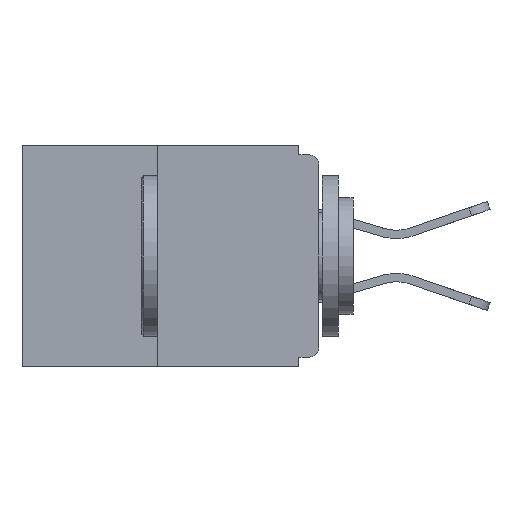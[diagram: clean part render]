
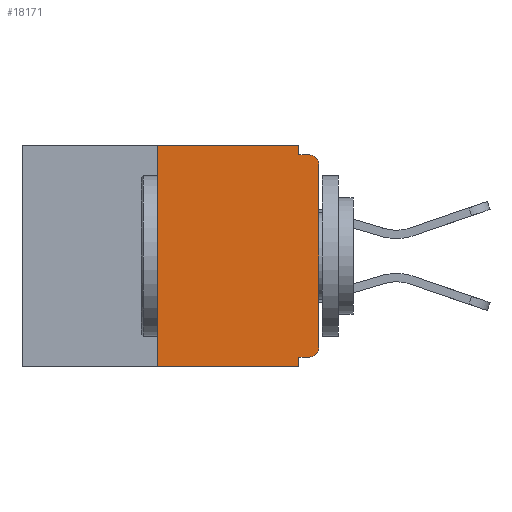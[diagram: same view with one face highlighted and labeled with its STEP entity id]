
A CAD part, left-side view. The second image highlights one B-rep face of the part: STEP entity #18171.
In plain terms, the highlighted planar face has unit normal (-1, 0, 0).
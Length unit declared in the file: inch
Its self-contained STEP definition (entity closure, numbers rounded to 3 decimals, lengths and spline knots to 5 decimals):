
#188 = CARTESIAN_POINT ( 'NONE',  ( 0., 0.031, 0. ) ) ;
#267 = DIRECTION ( 'NONE',  ( 0., 0., -1. ) ) ;
#459 = VECTOR ( 'NONE', #1966, 39.37008 ) ;
#1002 = VECTOR ( 'NONE', #4238, 39.37008 ) ;
#1060 = CARTESIAN_POINT ( 'NONE',  ( 0., 0., -0.015 ) ) ;
#1372 = CARTESIAN_POINT ( 'NONE',  ( 0., 0.46, -0.343 ) ) ;
#1966 = DIRECTION ( 'NONE',  ( 0., 0., 1. ) ) ;
#2070 = LINE ( 'NONE', #188, #21133 ) ;
#3008 = ORIENTED_EDGE ( 'NONE', *, *, #12980, .F. ) ;
#3172 = CARTESIAN_POINT ( 'NONE',  ( 0., 0.015, -0.313 ) ) ;
#3234 = DIRECTION ( 'NONE',  ( 0., 0., -1. ) ) ;
#3238 = CARTESIAN_POINT ( 'NONE',  ( 0., 0., 0. ) ) ;
#3423 = DIRECTION ( 'NONE',  ( -1., 0., 0. ) ) ;
#3539 = CARTESIAN_POINT ( 'NONE',  ( 0., 0.25, 0. ) ) ;
#3626 = CARTESIAN_POINT ( 'NONE',  ( 0., 0.25, 0. ) ) ;
#3891 = CARTESIAN_POINT ( 'NONE',  ( 0., 0.015, -0.328 ) ) ;
#4238 = DIRECTION ( 'NONE',  ( 0., -1., 0. ) ) ;
#4865 = VERTEX_POINT ( 'NONE', #9185 ) ;
#5002 = ORIENTED_EDGE ( 'NONE', *, *, #10056, .T. ) ;
#5117 = CARTESIAN_POINT ( 'NONE',  ( 0., 0.46, 0. ) ) ;
#5197 = CARTESIAN_POINT ( 'NONE',  ( 0., 0.031, -0.343 ) ) ;
#5343 = CARTESIAN_POINT ( 'NONE',  ( 0., 0.015, -0.03 ) ) ;
#6020 = EDGE_CURVE ( 'NONE', #9467, #15765, #13170, .T. ) ;
#6100 = VERTEX_POINT ( 'NONE', #13608 ) ;
#6797 = AXIS2_PLACEMENT_3D ( 'NONE', #5343, #9491, #20783 ) ;
#7282 = EDGE_CURVE ( 'NONE', #18928, #17246, #21570, .T. ) ;
#7414 = LINE ( 'NONE', #3238, #459 ) ;
#7417 = CARTESIAN_POINT ( 'NONE',  ( 0., 0., -0.03 ) ) ;
#8453 = EDGE_CURVE ( 'NONE', #17246, #20941, #2070, .T. ) ;
#8653 = ORIENTED_EDGE ( 'NONE', *, *, #7282, .F. ) ;
#8741 = CARTESIAN_POINT ( 'NONE',  ( 0., 0.015, -0.015 ) ) ;
#8863 = DIRECTION ( 'NONE',  ( 0., -1., 0. ) ) ;
#9185 = CARTESIAN_POINT ( 'NONE',  ( 0., 0., -0.313 ) ) ;
#9467 = VERTEX_POINT ( 'NONE', #7417 ) ;
#9491 = DIRECTION ( 'NONE',  ( -1., 0., 0. ) ) ;
#9983 = CARTESIAN_POINT ( 'NONE',  ( 0., 0.031, -0.015 ) ) ;
#10024 = VERTEX_POINT ( 'NONE', #20903 ) ;
#10034 = LINE ( 'NONE', #13744, #24865 ) ;
#10056 = EDGE_CURVE ( 'NONE', #4865, #9467, #7414, .T. ) ;
#10400 = LINE ( 'NONE', #3626, #17945 ) ;
#10794 = DIRECTION ( 'NONE',  ( 0., -1., 0. ) ) ;
#10860 = EDGE_LOOP ( 'NONE', ( #8653, #20169, #23829, #24696, #3008, #11767, #5002, #11875, #19360, #19040 ) ) ;
#11192 = EDGE_CURVE ( 'NONE', #20267, #18928, #10400, .T. ) ;
#11767 = ORIENTED_EDGE ( 'NONE', *, *, #15039, .T. ) ;
#11832 = DIRECTION ( 'NONE',  ( 0., 1., 0. ) ) ;
#11875 = ORIENTED_EDGE ( 'NONE', *, *, #6020, .T. ) ;
#12557 = CARTESIAN_POINT ( 'NONE',  ( 0., 0.031, 0. ) ) ;
#12980 = EDGE_CURVE ( 'NONE', #21988, #6100, #10034, .T. ) ;
#13128 = DIRECTION ( 'NONE',  ( 0., 0., -1. ) ) ;
#13146 = DIRECTION ( 'NONE',  ( 0., 0., -1. ) ) ;
#13170 = CIRCLE ( 'NONE', #6797, 0.015 ) ;
#13608 = CARTESIAN_POINT ( 'NONE',  ( 0., 0.031, -0.328 ) ) ;
#13621 = CARTESIAN_POINT ( 'NONE',  ( 0., 0.25, -0.343 ) ) ;
#13744 = CARTESIAN_POINT ( 'NONE',  ( 0., 0., -0.328 ) ) ;
#14809 = PLANE ( 'NONE',  #14847 ) ;
#14847 = AXIS2_PLACEMENT_3D ( 'NONE', #5117, #18619, #3234 ) ;
#15039 = EDGE_CURVE ( 'NONE', #21988, #4865, #18609, .T. ) ;
#15765 = VERTEX_POINT ( 'NONE', #8741 ) ;
#15998 = VECTOR ( 'NONE', #8863, 39.37008 ) ;
#16389 = VECTOR ( 'NONE', #13128, 39.37008 ) ;
#17226 = AXIS2_PLACEMENT_3D ( 'NONE', #3172, #3423, #13146 ) ;
#17246 = VERTEX_POINT ( 'NONE', #12557 ) ;
#17504 = LINE ( 'NONE', #1060, #15998 ) ;
#17906 = CARTESIAN_POINT ( 'NONE',  ( 0., 0.46, 0. ) ) ;
#17945 = VECTOR ( 'NONE', #24942, 39.37008 ) ;
#18108 = EDGE_CURVE ( 'NONE', #20267, #10024, #23680, .T. ) ;
#18171 = ADVANCED_FACE ( 'NONE', ( #22733 ), #14809, .F. ) ;
#18505 = VECTOR ( 'NONE', #10794, 39.37008 ) ;
#18609 = CIRCLE ( 'NONE', #17226, 0.015 ) ;
#18619 = DIRECTION ( 'NONE',  ( 1., 0., 0. ) ) ;
#18928 = VERTEX_POINT ( 'NONE', #3539 ) ;
#19040 = ORIENTED_EDGE ( 'NONE', *, *, #8453, .F. ) ;
#19284 = EDGE_CURVE ( 'NONE', #20941, #15765, #17504, .T. ) ;
#19360 = ORIENTED_EDGE ( 'NONE', *, *, #19284, .F. ) ;
#20169 = ORIENTED_EDGE ( 'NONE', *, *, #11192, .F. ) ;
#20267 = VERTEX_POINT ( 'NONE', #13621 ) ;
#20783 = DIRECTION ( 'NONE',  ( 0., 0., -1. ) ) ;
#20903 = CARTESIAN_POINT ( 'NONE',  ( 0., 0.031, -0.343 ) ) ;
#20941 = VERTEX_POINT ( 'NONE', #9983 ) ;
#21133 = VECTOR ( 'NONE', #267, 39.37008 ) ;
#21541 = LINE ( 'NONE', #5197, #16389 ) ;
#21570 = LINE ( 'NONE', #17906, #1002 ) ;
#21988 = VERTEX_POINT ( 'NONE', #3891 ) ;
#22733 = FACE_OUTER_BOUND ( 'NONE', #10860, .T. ) ;
#23054 = EDGE_CURVE ( 'NONE', #6100, #10024, #21541, .T. ) ;
#23680 = LINE ( 'NONE', #1372, #18505 ) ;
#23829 = ORIENTED_EDGE ( 'NONE', *, *, #18108, .T. ) ;
#24696 = ORIENTED_EDGE ( 'NONE', *, *, #23054, .F. ) ;
#24865 = VECTOR ( 'NONE', #11832, 39.37008 ) ;
#24942 = DIRECTION ( 'NONE',  ( 0., 0., 1. ) ) ;
